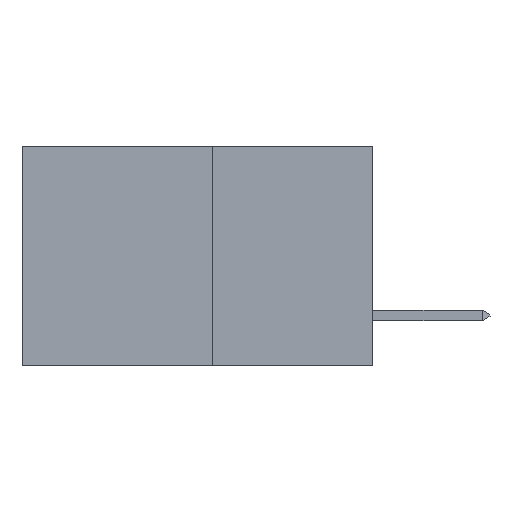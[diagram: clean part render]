
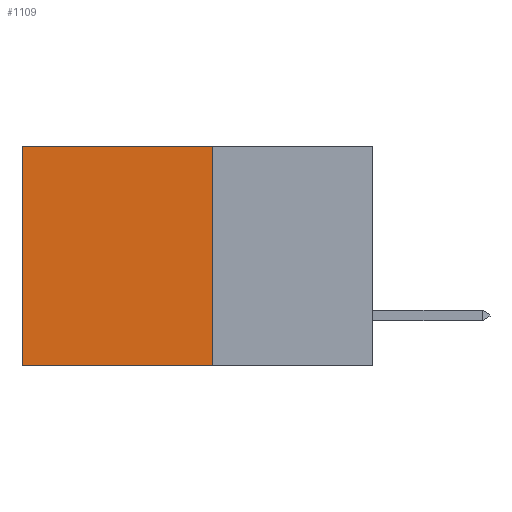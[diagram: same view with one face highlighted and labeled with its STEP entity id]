
A CAD part, left-side view. The second image highlights one B-rep face of the part: STEP entity #1109.
In plain terms, the highlighted planar face has unit normal (-1, 0, 0).
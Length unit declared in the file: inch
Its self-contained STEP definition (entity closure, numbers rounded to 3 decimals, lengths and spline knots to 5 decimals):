
#427 = DIRECTION ( 'NONE',  ( 0., 0., -1. ) ) ;
#1061 = EDGE_LOOP ( 'NONE', ( #10168, #19038, #5481, #15925 ) ) ;
#1109 = ADVANCED_FACE ( 'NONE', ( #12770 ), #4314, .F. ) ;
#1267 = CARTESIAN_POINT ( 'NONE',  ( 0.277, 0.27, -0.37 ) ) ;
#1781 = CARTESIAN_POINT ( 'NONE',  ( 0.277, 0.59, -0.37 ) ) ;
#1868 = EDGE_CURVE ( 'NONE', #15677, #18219, #15140, .T. ) ;
#2515 = EDGE_CURVE ( 'NONE', #15677, #13116, #11745, .T. ) ;
#2609 = VECTOR ( 'NONE', #10551, 39.37008 ) ;
#3159 = VECTOR ( 'NONE', #3395, 39.37008 ) ;
#3395 = DIRECTION ( 'NONE',  ( 0., 0., -1. ) ) ;
#3708 = CARTESIAN_POINT ( 'NONE',  ( 0.277, 0.27, -0.37 ) ) ;
#4314 = PLANE ( 'NONE',  #6715 ) ;
#4352 = CARTESIAN_POINT ( 'NONE',  ( 0.277, 0.27, -0.37 ) ) ;
#5435 = DIRECTION ( 'NONE',  ( 1., 0., 0. ) ) ;
#5481 = ORIENTED_EDGE ( 'NONE', *, *, #1868, .F. ) ;
#6715 = AXIS2_PLACEMENT_3D ( 'NONE', #3708, #5435, #18648 ) ;
#7969 = CARTESIAN_POINT ( 'NONE',  ( 0.277, 0.59, -0.37 ) ) ;
#8310 = CARTESIAN_POINT ( 'NONE',  ( 0.277, 0.27, -0.37 ) ) ;
#9010 = CARTESIAN_POINT ( 'NONE',  ( 0.277, 0.27, 0. ) ) ;
#9565 = EDGE_CURVE ( 'NONE', #13116, #11659, #19001, .T. ) ;
#10168 = ORIENTED_EDGE ( 'NONE', *, *, #9565, .T. ) ;
#10551 = DIRECTION ( 'NONE',  ( 0., 1., 0. ) ) ;
#11036 = VECTOR ( 'NONE', #427, 39.37008 ) ;
#11621 = CARTESIAN_POINT ( 'NONE',  ( 0.277, 0.59, 0. ) ) ;
#11659 = VERTEX_POINT ( 'NONE', #7969 ) ;
#11745 = LINE ( 'NONE', #9010, #15840 ) ;
#12149 = EDGE_CURVE ( 'NONE', #18219, #11659, #14457, .T. ) ;
#12749 = DIRECTION ( 'NONE',  ( 0., 1., 0. ) ) ;
#12770 = FACE_OUTER_BOUND ( 'NONE', #1061, .T. ) ;
#13116 = VERTEX_POINT ( 'NONE', #11621 ) ;
#14457 = LINE ( 'NONE', #1267, #2609 ) ;
#15140 = LINE ( 'NONE', #4352, #11036 ) ;
#15677 = VERTEX_POINT ( 'NONE', #18170 ) ;
#15840 = VECTOR ( 'NONE', #12749, 39.37008 ) ;
#15925 = ORIENTED_EDGE ( 'NONE', *, *, #2515, .T. ) ;
#18170 = CARTESIAN_POINT ( 'NONE',  ( 0.277, 0.27, 0. ) ) ;
#18219 = VERTEX_POINT ( 'NONE', #8310 ) ;
#18648 = DIRECTION ( 'NONE',  ( 0., 0., -1. ) ) ;
#19001 = LINE ( 'NONE', #1781, #3159 ) ;
#19038 = ORIENTED_EDGE ( 'NONE', *, *, #12149, .F. ) ;
